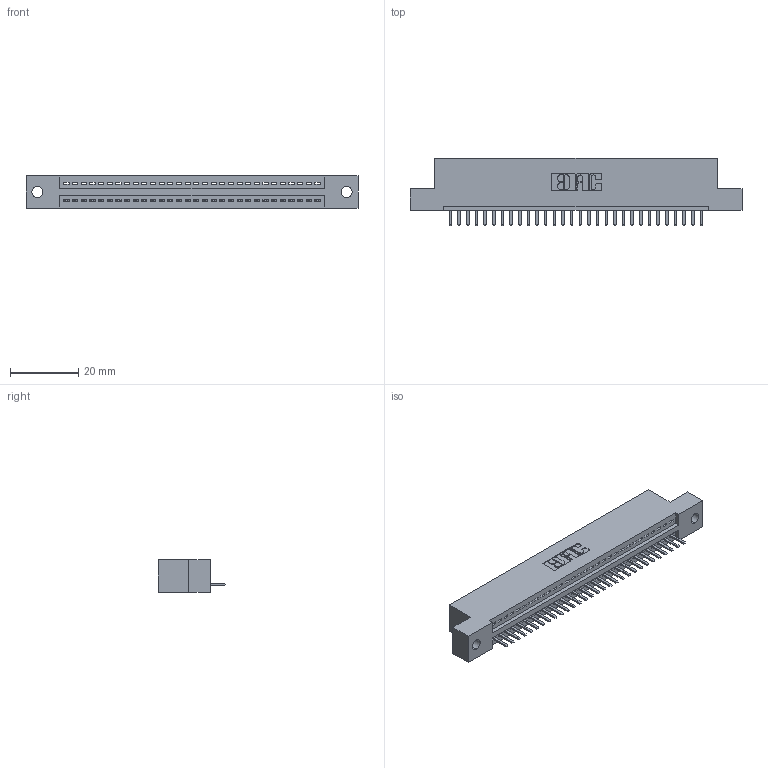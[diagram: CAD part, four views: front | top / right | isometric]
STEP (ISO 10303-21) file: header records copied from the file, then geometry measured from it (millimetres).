
FILE_DESCRIPTION (( 'STEP AP203' ), '1' );
FILE_NAME ('395-030-520-102.STEP', '2019-10-19T06:17:33', ( '' ), ( '' ), 'SwSTEP 2.0', 'SolidWorks 2016', '' );
FILE_SCHEMA (( 'CONFIG_CONTROL_DESIGN' ));
Length unit declared in the file: inch
Products named in the file (3): 345-292-001_345-293-120; 345 Part_Flush Mounting Lugs - 0.128 Dia; 395-030-520-102
Assembly tree (31 placements, depth 2):
  395-030-520-102
    345 Part_Flush Mounting Lugs - 0.128 Dia
    345-292-001_345-293-120  x30
Bounding box: 97.41 x 19.68 x 9.4 mm (x, y, z)
Volume: 9030.7 mm3; surface area: 11284.1 mm2
Topology: 31 solids, 31 shells, 1986 faces, 5861 edges, 3826 vertices
Faces by surface type: plane 1340, cylinder 646
Entity records: 24311 total; most frequent: CARTESIAN_POINT 4230, ORIENTED_EDGE 4182, DIRECTION 3699, EDGE_CURVE 2091, LINE 1835, VECTOR 1835, VERTEX_POINT 1390, AXIS2_PLACEMENT_3D 932
